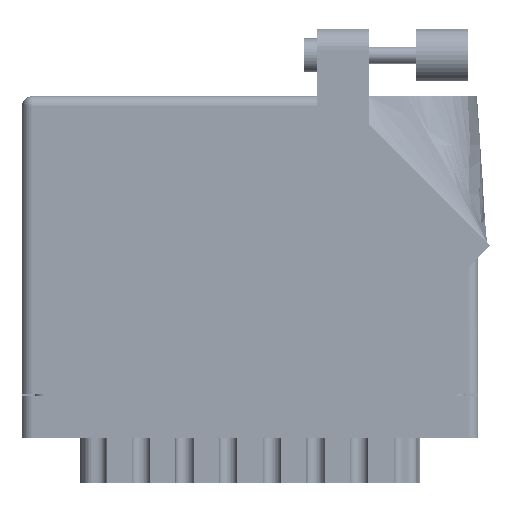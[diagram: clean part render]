
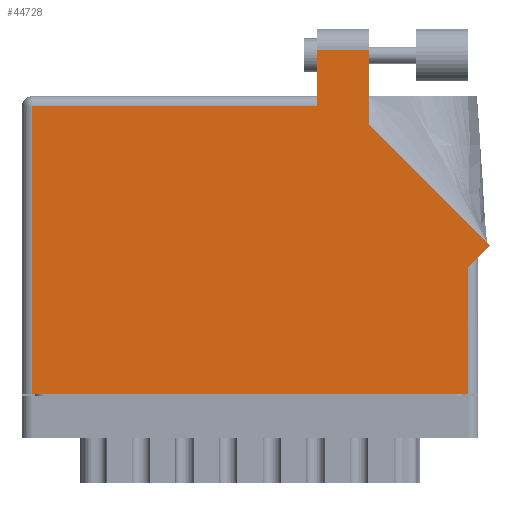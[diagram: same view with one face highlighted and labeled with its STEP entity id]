
A CAD part, front view. The second image highlights one B-rep face of the part: STEP entity #44728.
In plain terms, the highlighted face is planar.
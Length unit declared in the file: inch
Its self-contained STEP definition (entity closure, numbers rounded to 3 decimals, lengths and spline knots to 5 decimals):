
#1014 = ORIENTED_EDGE ( 'NONE', *, *, #2907, .T. ) ;
#1996 = CARTESIAN_POINT ( 'NONE',  ( 0.062, 0., 0. ) ) ;
#2075 = CARTESIAN_POINT ( 'NONE',  ( 2.78871, 0.88571, 0. ) ) ;
#2717 = LINE ( 'NONE', #1996, #68401 ) ;
#2902 = LINE ( 'NONE', #8462, #67886 ) ;
#2907 = EDGE_CURVE ( 'NONE', #51127, #3272, #11105, .T. ) ;
#3272 = VERTEX_POINT ( 'NONE', #27978 ) ;
#3740 = CARTESIAN_POINT ( 'NONE',  ( 2.718, 0.815, 0. ) ) ;
#6499 = EDGE_CURVE ( 'NONE', #3272, #48654, #68915, .T. ) ;
#7581 = DIRECTION ( 'NONE',  ( -1., 0., 0. ) ) ;
#7714 = CARTESIAN_POINT ( 'NONE',  ( 0.062, 0., 0. ) ) ;
#8462 = CARTESIAN_POINT ( 'NONE',  ( 0., 1.713, 0. ) ) ;
#11105 = LINE ( 'NONE', #34707, #25725 ) ;
#11276 = VERTEX_POINT ( 'NONE', #23828 ) ;
#13115 = FACE_OUTER_BOUND ( 'NONE', #28226, .T. ) ;
#13477 = DIRECTION ( 'NONE',  ( 0., 1., 0. ) ) ;
#14385 = CARTESIAN_POINT ( 'NONE',  ( 1.758, 1.775, 0. ) ) ;
#17725 = DIRECTION ( 'NONE',  ( 1., 0., 0. ) ) ;
#22591 = ORIENTED_EDGE ( 'NONE', *, *, #60429, .T. ) ;
#23484 = CARTESIAN_POINT ( 'NONE',  ( 2.065, 1.60942, 0. ) ) ;
#23828 = CARTESIAN_POINT ( 'NONE',  ( 1.758, 2.05, 0. ) ) ;
#24180 = CARTESIAN_POINT ( 'NONE',  ( 2.656, 0.815, 0. ) ) ;
#24912 = PLANE ( 'NONE',  #47986 ) ;
#25092 = ORIENTED_EDGE ( 'NONE', *, *, #6499, .T. ) ;
#25725 = VECTOR ( 'NONE', #17725, 39.37008 ) ;
#26372 = CARTESIAN_POINT ( 'NONE',  ( 2.656, 0.753, 0. ) ) ;
#27978 = CARTESIAN_POINT ( 'NONE',  ( 2.656, 0., 0. ) ) ;
#28003 = CARTESIAN_POINT ( 'NONE',  ( 0., 1.775, 0. ) ) ;
#28226 = EDGE_LOOP ( 'NONE', ( #52158, #22591, #50241, #30235, #45827, #1014, #25092, #72898, #38642 ) ) ;
#29752 = LINE ( 'NONE', #2075, #65374 ) ;
#30235 = ORIENTED_EDGE ( 'NONE', *, *, #38279, .T. ) ;
#34707 = CARTESIAN_POINT ( 'NONE',  ( 0., 0., 0. ) ) ;
#36899 = DIRECTION ( 'NONE',  ( 0., -1., 0. ) ) ;
#38279 = EDGE_CURVE ( 'NONE', #64667, #57013, #2902, .T. ) ;
#38642 = ORIENTED_EDGE ( 'NONE', *, *, #51828, .T. ) ;
#39451 = DIRECTION ( 'NONE',  ( 0., 0., -1. ) ) ;
#39545 = CARTESIAN_POINT ( 'NONE',  ( 2.065, 1.60942, 0. ) ) ;
#40113 = DIRECTION ( 'NONE',  ( 0., 1., 0. ) ) ;
#40410 = VERTEX_POINT ( 'NONE', #45553 ) ;
#40699 = VECTOR ( 'NONE', #50240, 39.37008 ) ;
#41556 = LINE ( 'NONE', #23484, #53513 ) ;
#43177 = LINE ( 'NONE', #14385, #67377 ) ;
#43560 = VECTOR ( 'NONE', #68272, 39.37008 ) ;
#44728 = ADVANCED_FACE ( 'NONE', ( #13115 ), #24912, .F. ) ;
#45553 = CARTESIAN_POINT ( 'NONE',  ( 2.78871, 0.88571, 0. ) ) ;
#45718 = CARTESIAN_POINT ( 'NONE',  ( 1.758, 2.05, 0. ) ) ;
#45827 = ORIENTED_EDGE ( 'NONE', *, *, #63450, .T. ) ;
#47413 = VERTEX_POINT ( 'NONE', #39545 ) ;
#47986 = AXIS2_PLACEMENT_3D ( 'NONE', #28003, #39451, #7581 ) ;
#48654 = VERTEX_POINT ( 'NONE', #26372 ) ;
#50240 = DIRECTION ( 'NONE',  ( 0.707, 0.707, 0. ) ) ;
#50241 = ORIENTED_EDGE ( 'NONE', *, *, #62023, .T. ) ;
#51127 = VERTEX_POINT ( 'NONE', #7714 ) ;
#51828 = EDGE_CURVE ( 'NONE', #40410, #47413, #29752, .T. ) ;
#52158 = ORIENTED_EDGE ( 'NONE', *, *, #70899, .T. ) ;
#52281 = DIRECTION ( 'NONE',  ( -0.707, 0.707, 0. ) ) ;
#53513 = VECTOR ( 'NONE', #40113, 39.37008 ) ;
#54332 = LINE ( 'NONE', #3740, #40699 ) ;
#55995 = VECTOR ( 'NONE', #13477, 39.37008 ) ;
#56047 = CARTESIAN_POINT ( 'NONE',  ( 1.758, 1.713, 0. ) ) ;
#57013 = VERTEX_POINT ( 'NONE', #70829 ) ;
#60429 = EDGE_CURVE ( 'NONE', #69573, #11276, #62721, .T. ) ;
#62023 = EDGE_CURVE ( 'NONE', #11276, #64667, #43177, .T. ) ;
#62721 = LINE ( 'NONE', #45718, #43560 ) ;
#63450 = EDGE_CURVE ( 'NONE', #57013, #51127, #2717, .T. ) ;
#64667 = VERTEX_POINT ( 'NONE', #56047 ) ;
#64963 = DIRECTION ( 'NONE',  ( -1., 0., 0. ) ) ;
#65374 = VECTOR ( 'NONE', #52281, 39.37008 ) ;
#66355 = CARTESIAN_POINT ( 'NONE',  ( 2.065, 2.05, 0. ) ) ;
#67377 = VECTOR ( 'NONE', #36899, 39.37008 ) ;
#67886 = VECTOR ( 'NONE', #64963, 39.37008 ) ;
#68272 = DIRECTION ( 'NONE',  ( -1., 0., 0. ) ) ;
#68401 = VECTOR ( 'NONE', #69603, 39.37008 ) ;
#68915 = LINE ( 'NONE', #24180, #55995 ) ;
#69573 = VERTEX_POINT ( 'NONE', #66355 ) ;
#69603 = DIRECTION ( 'NONE',  ( 0., -1., 0. ) ) ;
#70829 = CARTESIAN_POINT ( 'NONE',  ( 0.062, 1.713, 0. ) ) ;
#70899 = EDGE_CURVE ( 'NONE', #47413, #69573, #41556, .T. ) ;
#72260 = EDGE_CURVE ( 'NONE', #48654, #40410, #54332, .T. ) ;
#72898 = ORIENTED_EDGE ( 'NONE', *, *, #72260, .T. ) ;
